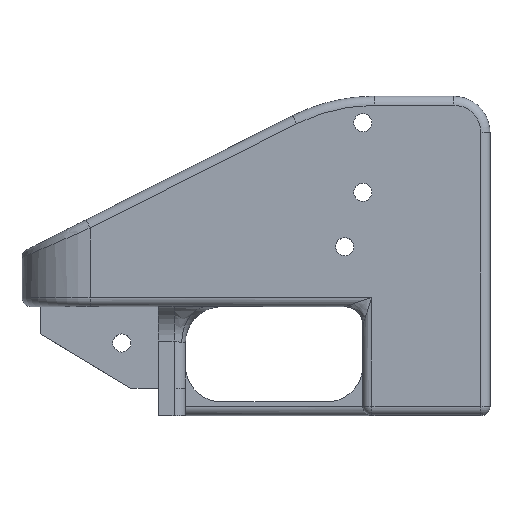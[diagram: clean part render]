
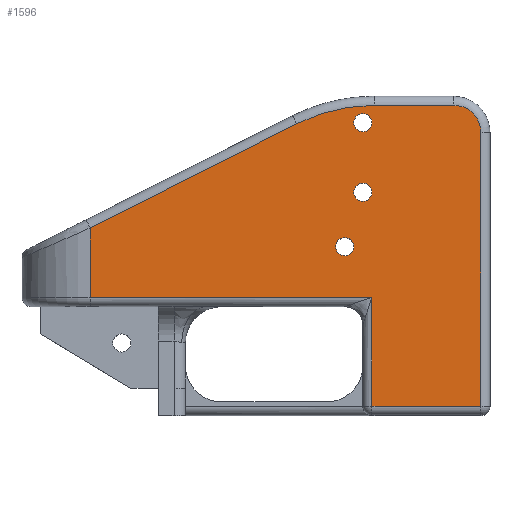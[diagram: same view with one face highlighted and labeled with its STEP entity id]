
A CAD part, top view. The second image highlights one B-rep face of the part: STEP entity #1596.
In plain terms, the highlighted planar face has unit normal (0, 0, 1).
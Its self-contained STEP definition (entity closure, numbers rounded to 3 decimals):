
#254 = DIRECTION ( 'NONE',  ( 1., 0., 0. ) ) ;
#266 = FACE_BOUND ( 'NONE', #4698, .T. ) ;
#288 = DIRECTION ( 'NONE',  ( -0.893, -0.45, 0. ) ) ;
#316 = CARTESIAN_POINT ( 'NONE',  ( 0., -27.94, 40.64 ) ) ;
#359 = EDGE_CURVE ( 'NONE', #1404, #1530, #3730, .T. ) ;
#398 = EDGE_CURVE ( 'NONE', #3027, #1225, #3483, .T. ) ;
#428 = ORIENTED_EDGE ( 'NONE', *, *, #698, .T. ) ;
#447 = VECTOR ( 'NONE', #785, 1000. ) ;
#466 = EDGE_CURVE ( 'NONE', #4128, #2467, #5168, .T. ) ;
#473 = EDGE_CURVE ( 'NONE', #4626, #3049, #3086, .T. ) ;
#500 = EDGE_CURVE ( 'NONE', #3049, #2419, #571, .T. ) ;
#509 = EDGE_CURVE ( 'NONE', #2419, #3339, #1651, .T. ) ;
#533 = EDGE_CURVE ( 'NONE', #3339, #1367, #2536, .T. ) ;
#542 = EDGE_CURVE ( 'NONE', #1367, #2089, #2394, .T. ) ;
#569 = EDGE_CURVE ( 'NONE', #2089, #1055, #4246, .T. ) ;
#571 = LINE ( 'NONE', #1165, #447 ) ;
#576 = PLANE ( 'NONE',  #2114 ) ;
#623 = EDGE_CURVE ( 'NONE', #1055, #4760, #4951, .T. ) ;
#628 = CARTESIAN_POINT ( 'NONE',  ( -110.744, 22.572, 40.64 ) ) ;
#698 = EDGE_CURVE ( 'NONE', #4760, #2555, #999, .T. ) ;
#781 = CARTESIAN_POINT ( 'NONE',  ( -33.02, -27.94, 40.64 ) ) ;
#785 = DIRECTION ( 'NONE',  ( 0., -1., 0. ) ) ;
#797 = ORIENTED_EDGE ( 'NONE', *, *, #500, .T. ) ;
#800 = VECTOR ( 'NONE', #4512, 1000. ) ;
#957 = CARTESIAN_POINT ( 'NONE',  ( -43.18, 16.764, 40.64 ) ) ;
#999 = LINE ( 'NONE', #628, #5414 ) ;
#1055 = VERTEX_POINT ( 'NONE', #4684 ) ;
#1100 = CARTESIAN_POINT ( 'NONE',  ( -33.02, 51.46, 40.64 ) ) ;
#1120 = CARTESIAN_POINT ( 'NONE',  ( -111.887, 0., 40.64 ) ) ;
#1165 = CARTESIAN_POINT ( 'NONE',  ( -33.02, 0., 40.64 ) ) ;
#1178 = CARTESIAN_POINT ( 'NONE',  ( -33.02, 2.54, 40.64 ) ) ;
#1225 = VERTEX_POINT ( 'NONE', #3190 ) ;
#1364 = DIRECTION ( 'NONE',  ( 1., 0., 0. ) ) ;
#1367 = VERTEX_POINT ( 'NONE', #1663 ) ;
#1380 = VECTOR ( 'NONE', #5132, 1000. ) ;
#1404 = VERTEX_POINT ( 'NONE', #2976 ) ;
#1530 = VERTEX_POINT ( 'NONE', #957 ) ;
#1567 = DIRECTION ( 'NONE',  ( 0., 0., 1. ) ) ;
#1568 = DIRECTION ( 'NONE',  ( 0., -1., 0. ) ) ;
#1576 = CARTESIAN_POINT ( 'NONE',  ( -40.64, 16.764, 40.64 ) ) ;
#1590 = CARTESIAN_POINT ( 'NONE',  ( -35.56, 51.46, 40.64 ) ) ;
#1596 = ADVANCED_FACE ( 'NONE', ( #2513, #266, #4611, #3517 ), #576, .T. ) ;
#1612 = DIRECTION ( 'NONE',  ( 1., 0., 0. ) ) ;
#1651 = LINE ( 'NONE', #316, #2674 ) ;
#1663 = CARTESIAN_POINT ( 'NONE',  ( -2.54, 48.666, 40.64 ) ) ;
#1701 = ORIENTED_EDGE ( 'NONE', *, *, #3520, .F. ) ;
#1729 = DIRECTION ( 'NONE',  ( 1., 0., 0. ) ) ;
#1748 = CARTESIAN_POINT ( 'NONE',  ( -35.56, 2.54, 40.64 ) ) ;
#1768 = ORIENTED_EDGE ( 'NONE', *, *, #466, .F. ) ;
#1774 = AXIS2_PLACEMENT_3D ( 'NONE', #1590, #1567, #1364 ) ;
#1817 = CARTESIAN_POINT ( 'NONE',  ( -35.56, 51.46, 40.64 ) ) ;
#1837 = ORIENTED_EDGE ( 'NONE', *, *, #5478, .T. ) ;
#1872 = EDGE_LOOP ( 'NONE', ( #4369, #2412 ) ) ;
#2028 = DIRECTION ( 'NONE',  ( 1., 0., 0. ) ) ;
#2089 = VERTEX_POINT ( 'NONE', #4413 ) ;
#2107 = AXIS2_PLACEMENT_3D ( 'NONE', #4152, #4125, #4104 ) ;
#2114 = AXIS2_PLACEMENT_3D ( 'NONE', #4003, #5302, #4878 ) ;
#2155 = EDGE_LOOP ( 'NONE', ( #1768, #1701 ) ) ;
#2262 = DIRECTION ( 'NONE',  ( 1., 0., 0. ) ) ;
#2331 = DIRECTION ( 'NONE',  ( 0., 0., 1. ) ) ;
#2390 = AXIS2_PLACEMENT_3D ( 'NONE', #2851, #2833, #1729 ) ;
#2394 = CIRCLE ( 'NONE', #2107, 7.62 ) ;
#2412 = ORIENTED_EDGE ( 'NONE', *, *, #4750, .F. ) ;
#2419 = VERTEX_POINT ( 'NONE', #781 ) ;
#2446 = ORIENTED_EDGE ( 'NONE', *, *, #509, .T. ) ;
#2467 = VERTEX_POINT ( 'NONE', #4280 ) ;
#2513 = FACE_BOUND ( 'NONE', #1872, .T. ) ;
#2536 = LINE ( 'NONE', #5114, #1380 ) ;
#2555 = VERTEX_POINT ( 'NONE', #5149 ) ;
#2674 = VECTOR ( 'NONE', #254, 1000. ) ;
#2779 = EDGE_CURVE ( 'NONE', #1225, #3027, #4551, .T. ) ;
#2833 = DIRECTION ( 'NONE',  ( 0., 0., 1. ) ) ;
#2851 = CARTESIAN_POINT ( 'NONE',  ( -32.373, 8.026, 40.64 ) ) ;
#2950 = VECTOR ( 'NONE', #1612, 1000. ) ;
#2959 = CARTESIAN_POINT ( 'NONE',  ( -2.54, -27.94, 40.64 ) ) ;
#2976 = CARTESIAN_POINT ( 'NONE',  ( -38.1, 16.764, 40.64 ) ) ;
#3027 = VERTEX_POINT ( 'NONE', #3340 ) ;
#3040 = AXIS2_PLACEMENT_3D ( 'NONE', #1817, #4778, #2262 ) ;
#3049 = VERTEX_POINT ( 'NONE', #1178 ) ;
#3086 = LINE ( 'NONE', #1748, #2950 ) ;
#3190 = CARTESIAN_POINT ( 'NONE',  ( -38.1, 32.004, 40.64 ) ) ;
#3204 = CARTESIAN_POINT ( 'NONE',  ( -111.887, 2.54, 40.64 ) ) ;
#3242 = AXIS2_PLACEMENT_3D ( 'NONE', #1576, #4556, #2028 ) ;
#3339 = VERTEX_POINT ( 'NONE', #2959 ) ;
#3340 = CARTESIAN_POINT ( 'NONE',  ( -33.02, 32.004, 40.64 ) ) ;
#3425 = DIRECTION ( 'NONE',  ( 1., 0., 0. ) ) ;
#3462 = DIRECTION ( 'NONE',  ( 0., 0., 1. ) ) ;
#3483 = CIRCLE ( 'NONE', #5282, 2.54 ) ;
#3484 = CARTESIAN_POINT ( 'NONE',  ( -35.56, 32.004, 40.64 ) ) ;
#3486 = CARTESIAN_POINT ( 'NONE',  ( -32.373, 56.286, 40.64 ) ) ;
#3517 = FACE_OUTER_BOUND ( 'NONE', #3551, .T. ) ;
#3520 = EDGE_CURVE ( 'NONE', #2467, #4128, #5458, .T. ) ;
#3539 = LINE ( 'NONE', #1120, #4513 ) ;
#3544 = ORIENTED_EDGE ( 'NONE', *, *, #623, .T. ) ;
#3551 = EDGE_LOOP ( 'NONE', ( #4941, #797, #2446, #4240, #5103, #3781, #3544, #428, #1837 ) ) ;
#3730 = CIRCLE ( 'NONE', #3983, 2.54 ) ;
#3781 = ORIENTED_EDGE ( 'NONE', *, *, #569, .T. ) ;
#3799 = AXIS2_PLACEMENT_3D ( 'NONE', #4844, #2331, #5271 ) ;
#3805 = ORIENTED_EDGE ( 'NONE', *, *, #2779, .F. ) ;
#3983 = AXIS2_PLACEMENT_3D ( 'NONE', #4548, #4317, #4298 ) ;
#4003 = CARTESIAN_POINT ( 'NONE',  ( 0., 0., 40.64 ) ) ;
#4104 = DIRECTION ( 'NONE',  ( 1., 0., 0. ) ) ;
#4125 = DIRECTION ( 'NONE',  ( 0., 0., 1. ) ) ;
#4128 = VERTEX_POINT ( 'NONE', #1100 ) ;
#4152 = CARTESIAN_POINT ( 'NONE',  ( -10.16, 48.666, 40.64 ) ) ;
#4240 = ORIENTED_EDGE ( 'NONE', *, *, #533, .T. ) ;
#4246 = LINE ( 'NONE', #3486, #800 ) ;
#4280 = CARTESIAN_POINT ( 'NONE',  ( -38.1, 51.46, 40.64 ) ) ;
#4298 = DIRECTION ( 'NONE',  ( 1., 0., 0. ) ) ;
#4317 = DIRECTION ( 'NONE',  ( 0., 0., 1. ) ) ;
#4369 = ORIENTED_EDGE ( 'NONE', *, *, #359, .F. ) ;
#4413 = CARTESIAN_POINT ( 'NONE',  ( -10.16, 56.286, 40.64 ) ) ;
#4512 = DIRECTION ( 'NONE',  ( -1., 0., 0. ) ) ;
#4513 = VECTOR ( 'NONE', #1568, 1000. ) ;
#4548 = CARTESIAN_POINT ( 'NONE',  ( -40.64, 16.764, 40.64 ) ) ;
#4551 = CIRCLE ( 'NONE', #3799, 2.54 ) ;
#4556 = DIRECTION ( 'NONE',  ( 0., 0., 1. ) ) ;
#4611 = FACE_BOUND ( 'NONE', #2155, .T. ) ;
#4626 = VERTEX_POINT ( 'NONE', #3204 ) ;
#4684 = CARTESIAN_POINT ( 'NONE',  ( -32.373, 56.286, 40.64 ) ) ;
#4698 = EDGE_LOOP ( 'NONE', ( #5412, #3805 ) ) ;
#4750 = EDGE_CURVE ( 'NONE', #1530, #1404, #5299, .T. ) ;
#4760 = VERTEX_POINT ( 'NONE', #4952 ) ;
#4778 = DIRECTION ( 'NONE',  ( 0., 0., 1. ) ) ;
#4844 = CARTESIAN_POINT ( 'NONE',  ( -35.56, 32.004, 40.64 ) ) ;
#4878 = DIRECTION ( 'NONE',  ( 1., 0., 0. ) ) ;
#4941 = ORIENTED_EDGE ( 'NONE', *, *, #473, .T. ) ;
#4951 = CIRCLE ( 'NONE', #2390, 48.26 ) ;
#4952 = CARTESIAN_POINT ( 'NONE',  ( -54.092, 51.123, 40.64 ) ) ;
#5103 = ORIENTED_EDGE ( 'NONE', *, *, #542, .T. ) ;
#5114 = CARTESIAN_POINT ( 'NONE',  ( -2.54, 48.666, 40.64 ) ) ;
#5132 = DIRECTION ( 'NONE',  ( 0., 1., 0. ) ) ;
#5149 = CARTESIAN_POINT ( 'NONE',  ( -111.887, 21.996, 40.64 ) ) ;
#5168 = CIRCLE ( 'NONE', #1774, 2.54 ) ;
#5271 = DIRECTION ( 'NONE',  ( 1., 0., 0. ) ) ;
#5282 = AXIS2_PLACEMENT_3D ( 'NONE', #3484, #3462, #3425 ) ;
#5299 = CIRCLE ( 'NONE', #3242, 2.54 ) ;
#5302 = DIRECTION ( 'NONE',  ( 0., 0., 1. ) ) ;
#5412 = ORIENTED_EDGE ( 'NONE', *, *, #398, .F. ) ;
#5414 = VECTOR ( 'NONE', #288, 1000. ) ;
#5458 = CIRCLE ( 'NONE', #3040, 2.54 ) ;
#5478 = EDGE_CURVE ( 'NONE', #2555, #4626, #3539, .T. ) ;
